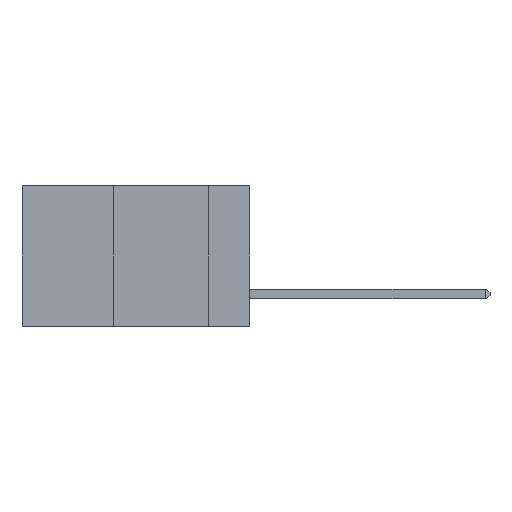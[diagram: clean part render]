
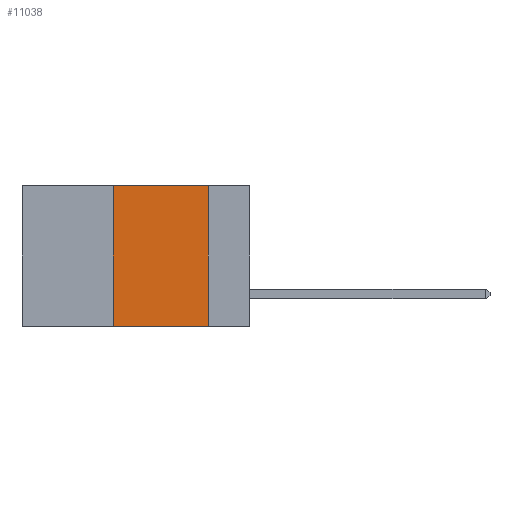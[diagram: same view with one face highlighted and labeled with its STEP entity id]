
A CAD part, left-side view. The second image highlights one B-rep face of the part: STEP entity #11038.
In plain terms, the highlighted planar face has unit normal (-1, 0, 0).
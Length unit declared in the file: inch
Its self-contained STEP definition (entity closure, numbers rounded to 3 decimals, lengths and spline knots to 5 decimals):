
#313 = LINE ( 'NONE', #7825, #5411 ) ;
#706 = ORIENTED_EDGE ( 'NONE', *, *, #10693, .F. ) ;
#1067 = DIRECTION ( 'NONE',  ( 0., 0., -1. ) ) ;
#1116 = VERTEX_POINT ( 'NONE', #12037 ) ;
#1393 = LINE ( 'NONE', #4443, #5869 ) ;
#1618 = DIRECTION ( 'NONE',  ( 0., 0., -1. ) ) ;
#1785 = CARTESIAN_POINT ( 'NONE',  ( 0., 0.36, 0. ) ) ;
#2920 = DIRECTION ( 'NONE',  ( 0., -1., 0. ) ) ;
#3248 = VECTOR ( 'NONE', #1067, 39.37008 ) ;
#3371 = VERTEX_POINT ( 'NONE', #12206 ) ;
#3412 = DIRECTION ( 'NONE',  ( 0., -1., 0. ) ) ;
#3801 = EDGE_CURVE ( 'NONE', #11468, #5309, #1393, .T. ) ;
#4237 = AXIS2_PLACEMENT_3D ( 'NONE', #5638, #7622, #1618 ) ;
#4272 = CARTESIAN_POINT ( 'NONE',  ( 0., 0.36, -0.37 ) ) ;
#4443 = CARTESIAN_POINT ( 'NONE',  ( 0., 0.6, -0.37 ) ) ;
#4564 = VECTOR ( 'NONE', #12211, 39.37008 ) ;
#5309 = VERTEX_POINT ( 'NONE', #5549 ) ;
#5411 = VECTOR ( 'NONE', #2920, 39.37008 ) ;
#5508 = LINE ( 'NONE', #1785, #4564 ) ;
#5549 = CARTESIAN_POINT ( 'NONE',  ( 0., 0.11, -0.37 ) ) ;
#5638 = CARTESIAN_POINT ( 'NONE',  ( 0., 0.6, 0. ) ) ;
#5869 = VECTOR ( 'NONE', #3412, 39.37008 ) ;
#5987 = ORIENTED_EDGE ( 'NONE', *, *, #11831, .F. ) ;
#7109 = CARTESIAN_POINT ( 'NONE',  ( 0., 0.11, 0. ) ) ;
#7622 = DIRECTION ( 'NONE',  ( 1., 0., 0. ) ) ;
#7701 = ORIENTED_EDGE ( 'NONE', *, *, #8280, .F. ) ;
#7825 = CARTESIAN_POINT ( 'NONE',  ( 0., 0.6, 0. ) ) ;
#8165 = ORIENTED_EDGE ( 'NONE', *, *, #3801, .T. ) ;
#8280 = EDGE_CURVE ( 'NONE', #3371, #5309, #10192, .T. ) ;
#9037 = FACE_OUTER_BOUND ( 'NONE', #11530, .T. ) ;
#10192 = LINE ( 'NONE', #7109, #3248 ) ;
#10229 = PLANE ( 'NONE',  #4237 ) ;
#10693 = EDGE_CURVE ( 'NONE', #1116, #3371, #313, .T. ) ;
#11038 = ADVANCED_FACE ( 'NONE', ( #9037 ), #10229, .F. ) ;
#11468 = VERTEX_POINT ( 'NONE', #4272 ) ;
#11530 = EDGE_LOOP ( 'NONE', ( #7701, #706, #5987, #8165 ) ) ;
#11831 = EDGE_CURVE ( 'NONE', #11468, #1116, #5508, .T. ) ;
#12037 = CARTESIAN_POINT ( 'NONE',  ( 0., 0.36, 0. ) ) ;
#12206 = CARTESIAN_POINT ( 'NONE',  ( 0., 0.11, 0. ) ) ;
#12211 = DIRECTION ( 'NONE',  ( 0., 0., 1. ) ) ;
